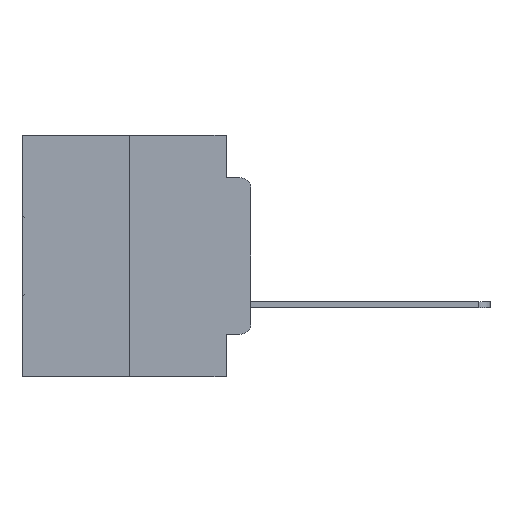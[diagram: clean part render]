
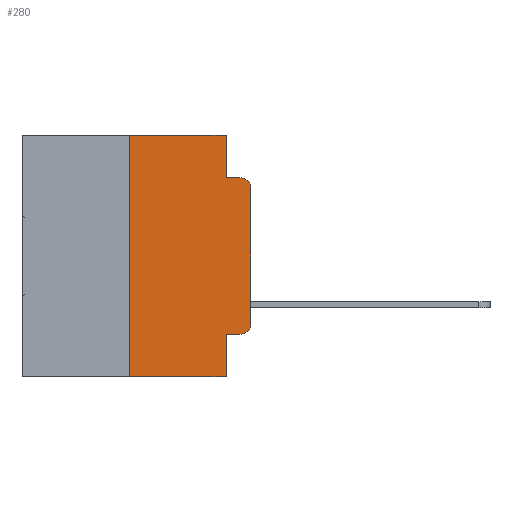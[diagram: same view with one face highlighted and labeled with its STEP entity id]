
A CAD part, left-side view. The second image highlights one B-rep face of the part: STEP entity #280.
In plain terms, the highlighted planar face has unit normal (-1, 0, 0).
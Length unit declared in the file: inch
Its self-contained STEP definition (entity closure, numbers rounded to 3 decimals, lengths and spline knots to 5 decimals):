
#280 = ADVANCED_FACE ( 'NONE', ( #16246 ), #21843, .F. ) ;
#1808 = CARTESIAN_POINT ( 'NONE',  ( 0., 0.051, -0.4115 ) ) ;
#3337 = CARTESIAN_POINT ( 'NONE',  ( 0., 0.02, -0.1085 ) ) ;
#3819 = CARTESIAN_POINT ( 'NONE',  ( 0., 0.051, -0.0885 ) ) ;
#4117 = CARTESIAN_POINT ( 'NONE',  ( 0., 0.02, -0.0885 ) ) ;
#4145 = ORIENTED_EDGE ( 'NONE', *, *, #8085, .T. ) ;
#4674 = LINE ( 'NONE', #19668, #23922 ) ;
#4900 = ORIENTED_EDGE ( 'NONE', *, *, #12317, .T. ) ;
#5317 = ORIENTED_EDGE ( 'NONE', *, *, #13706, .F. ) ;
#5839 = CIRCLE ( 'NONE', #18047, 0.02 ) ;
#5894 = DIRECTION ( 'NONE',  ( 0., 0., -1. ) ) ;
#6163 = AXIS2_PLACEMENT_3D ( 'NONE', #22656, #7588, #25056 ) ;
#6406 = EDGE_CURVE ( 'NONE', #17394, #23107, #28149, .T. ) ;
#6884 = CARTESIAN_POINT ( 'NONE',  ( 0., 0.051, 0. ) ) ;
#7251 = DIRECTION ( 'NONE',  ( 0., 0., 1. ) ) ;
#7588 = DIRECTION ( 'NONE',  ( -1., 0., 0. ) ) ;
#8085 = EDGE_CURVE ( 'NONE', #10404, #17394, #29557, .T. ) ;
#8147 = VERTEX_POINT ( 'NONE', #12106 ) ;
#8909 = CARTESIAN_POINT ( 'NONE',  ( 0., 0., -0.3915 ) ) ;
#8978 = EDGE_CURVE ( 'NONE', #25238, #18355, #5839, .T. ) ;
#9358 = CARTESIAN_POINT ( 'NONE',  ( 0., 0.051, 0. ) ) ;
#9508 = VECTOR ( 'NONE', #17314, 39.37008 ) ;
#10104 = ORIENTED_EDGE ( 'NONE', *, *, #12513, .F. ) ;
#10404 = VERTEX_POINT ( 'NONE', #31594 ) ;
#11499 = VECTOR ( 'NONE', #14447, 39.37008 ) ;
#12106 = CARTESIAN_POINT ( 'NONE',  ( 0., 0.051, -0.5 ) ) ;
#12317 = EDGE_CURVE ( 'NONE', #23107, #25238, #27037, .T. ) ;
#12513 = EDGE_CURVE ( 'NONE', #10404, #8147, #29678, .T. ) ;
#12840 = VERTEX_POINT ( 'NONE', #9358 ) ;
#13647 = EDGE_CURVE ( 'NONE', #14888, #8147, #21228, .T. ) ;
#13706 = EDGE_CURVE ( 'NONE', #22874, #12840, #4674, .T. ) ;
#13779 = CARTESIAN_POINT ( 'NONE',  ( 0., 0.473, 0. ) ) ;
#13899 = VECTOR ( 'NONE', #7251, 39.37008 ) ;
#14020 = ORIENTED_EDGE ( 'NONE', *, *, #19702, .F. ) ;
#14447 = DIRECTION ( 'NONE',  ( 0., 0., 1. ) ) ;
#14773 = CARTESIAN_POINT ( 'NONE',  ( 0., 0.051, -0.0885 ) ) ;
#14811 = VERTEX_POINT ( 'NONE', #3819 ) ;
#14888 = VERTEX_POINT ( 'NONE', #19266 ) ;
#15398 = LINE ( 'NONE', #14773, #9508 ) ;
#15408 = DIRECTION ( 'NONE',  ( 0., 0., -1. ) ) ;
#15515 = CARTESIAN_POINT ( 'NONE',  ( 0., 0.051, 0. ) ) ;
#16246 = FACE_OUTER_BOUND ( 'NONE', #27491, .T. ) ;
#16516 = VECTOR ( 'NONE', #24461, 39.37008 ) ;
#16789 = DIRECTION ( 'NONE',  ( 1., 0., 0. ) ) ;
#17314 = DIRECTION ( 'NONE',  ( 0., -1., 0. ) ) ;
#17394 = VERTEX_POINT ( 'NONE', #17874 ) ;
#17443 = LINE ( 'NONE', #31588, #11499 ) ;
#17874 = CARTESIAN_POINT ( 'NONE',  ( 0., 0.02, -0.4115 ) ) ;
#18047 = AXIS2_PLACEMENT_3D ( 'NONE', #3337, #20971, #5894 ) ;
#18061 = CARTESIAN_POINT ( 'NONE',  ( 0., 0.25, 0. ) ) ;
#18355 = VERTEX_POINT ( 'NONE', #4117 ) ;
#19266 = CARTESIAN_POINT ( 'NONE',  ( 0., 0.25, -0.5 ) ) ;
#19668 = CARTESIAN_POINT ( 'NONE',  ( 0., 0.473, 0. ) ) ;
#19702 = EDGE_CURVE ( 'NONE', #14811, #18355, #15398, .T. ) ;
#19942 = ORIENTED_EDGE ( 'NONE', *, *, #6406, .T. ) ;
#20465 = VECTOR ( 'NONE', #24215, 39.37008 ) ;
#20971 = DIRECTION ( 'NONE',  ( -1., 0., 0. ) ) ;
#21080 = ORIENTED_EDGE ( 'NONE', *, *, #13647, .T. ) ;
#21228 = LINE ( 'NONE', #26702, #20465 ) ;
#21843 = PLANE ( 'NONE',  #25291 ) ;
#22503 = VECTOR ( 'NONE', #15408, 39.37008 ) ;
#22621 = DIRECTION ( 'NONE',  ( 0., 0., -1. ) ) ;
#22656 = CARTESIAN_POINT ( 'NONE',  ( 0., 0.02, -0.3915 ) ) ;
#22874 = VERTEX_POINT ( 'NONE', #18061 ) ;
#23107 = VERTEX_POINT ( 'NONE', #8909 ) ;
#23509 = VECTOR ( 'NONE', #24390, 39.37008 ) ;
#23922 = VECTOR ( 'NONE', #31657, 39.37008 ) ;
#24215 = DIRECTION ( 'NONE',  ( 0., -1., 0. ) ) ;
#24390 = DIRECTION ( 'NONE',  ( 0., 0., -1. ) ) ;
#24461 = DIRECTION ( 'NONE',  ( 0., -1., 0. ) ) ;
#25056 = DIRECTION ( 'NONE',  ( 0., 0., -1. ) ) ;
#25229 = EDGE_CURVE ( 'NONE', #12840, #14811, #29146, .T. ) ;
#25238 = VERTEX_POINT ( 'NONE', #26687 ) ;
#25291 = AXIS2_PLACEMENT_3D ( 'NONE', #13779, #16789, #22621 ) ;
#26392 = ORIENTED_EDGE ( 'NONE', *, *, #8978, .T. ) ;
#26687 = CARTESIAN_POINT ( 'NONE',  ( 0., 0., -0.1085 ) ) ;
#26702 = CARTESIAN_POINT ( 'NONE',  ( 0., 0.473, -0.5 ) ) ;
#26787 = ORIENTED_EDGE ( 'NONE', *, *, #32284, .F. ) ;
#27037 = LINE ( 'NONE', #31909, #13899 ) ;
#27491 = EDGE_LOOP ( 'NONE', ( #4900, #26392, #14020, #27917, #5317, #26787, #21080, #10104, #4145, #19942 ) ) ;
#27917 = ORIENTED_EDGE ( 'NONE', *, *, #25229, .F. ) ;
#28149 = CIRCLE ( 'NONE', #6163, 0.02 ) ;
#29146 = LINE ( 'NONE', #6884, #23509 ) ;
#29557 = LINE ( 'NONE', #1808, #16516 ) ;
#29678 = LINE ( 'NONE', #15515, #22503 ) ;
#31588 = CARTESIAN_POINT ( 'NONE',  ( 0., 0.25, 0. ) ) ;
#31594 = CARTESIAN_POINT ( 'NONE',  ( 0., 0.051, -0.4115 ) ) ;
#31657 = DIRECTION ( 'NONE',  ( 0., -1., 0. ) ) ;
#31909 = CARTESIAN_POINT ( 'NONE',  ( 0., 0., 0. ) ) ;
#32284 = EDGE_CURVE ( 'NONE', #14888, #22874, #17443, .T. ) ;
